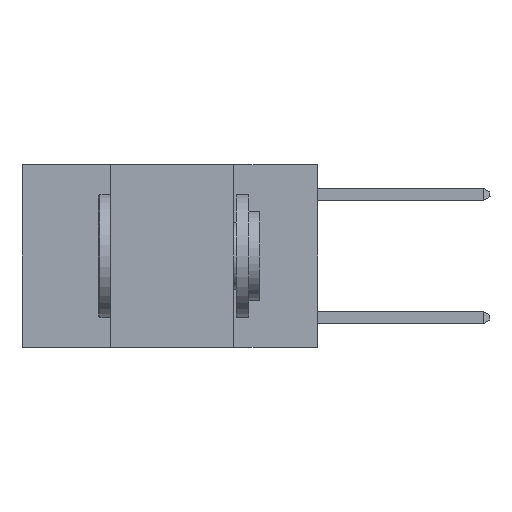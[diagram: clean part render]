
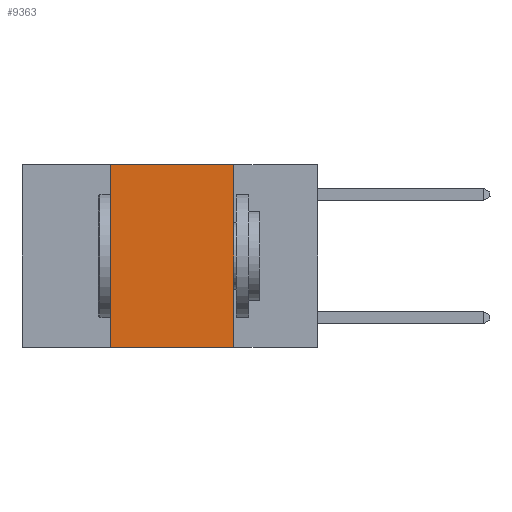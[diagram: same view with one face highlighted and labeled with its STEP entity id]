
A CAD part, left-side view. The second image highlights one B-rep face of the part: STEP entity #9363.
In plain terms, the highlighted planar face has unit normal (-1, 0, 0).
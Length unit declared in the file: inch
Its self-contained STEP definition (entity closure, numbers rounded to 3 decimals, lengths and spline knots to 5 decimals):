
#421 = DIRECTION ( 'NONE',  ( 0., 0., -1. ) ) ;
#460 = ORIENTED_EDGE ( 'NONE', *, *, #572, .F. ) ;
#572 = EDGE_CURVE ( 'NONE', #6092, #12067, #3695, .T. ) ;
#1472 = LINE ( 'NONE', #5365, #6991 ) ;
#2053 = CARTESIAN_POINT ( 'NONE',  ( 0., 0.17, -0.37 ) ) ;
#2144 = PLANE ( 'NONE',  #12619 ) ;
#2571 = LINE ( 'NONE', #11408, #7800 ) ;
#3351 = VECTOR ( 'NONE', #421, 39.37008 ) ;
#3398 = VERTEX_POINT ( 'NONE', #11470 ) ;
#3695 = LINE ( 'NONE', #10714, #3351 ) ;
#4326 = DIRECTION ( 'NONE',  ( 1., 0., 0. ) ) ;
#5365 = CARTESIAN_POINT ( 'NONE',  ( 0., 0.42, 0. ) ) ;
#5395 = CARTESIAN_POINT ( 'NONE',  ( 0., 0.6, 0. ) ) ;
#5823 = DIRECTION ( 'NONE',  ( 0., -1., 0. ) ) ;
#6092 = VERTEX_POINT ( 'NONE', #9779 ) ;
#6991 = VECTOR ( 'NONE', #14229, 39.37008 ) ;
#7011 = CARTESIAN_POINT ( 'NONE',  ( 0., 0.42, 0. ) ) ;
#7800 = VECTOR ( 'NONE', #5823, 39.37008 ) ;
#8449 = EDGE_LOOP ( 'NONE', ( #460, #9963, #9707, #10743 ) ) ;
#8505 = EDGE_CURVE ( 'NONE', #3398, #10678, #1472, .T. ) ;
#8851 = LINE ( 'NONE', #12015, #11480 ) ;
#9363 = ADVANCED_FACE ( 'NONE', ( #12208 ), #2144, .F. ) ;
#9707 = ORIENTED_EDGE ( 'NONE', *, *, #8505, .F. ) ;
#9708 = EDGE_CURVE ( 'NONE', #10678, #6092, #8851, .T. ) ;
#9779 = CARTESIAN_POINT ( 'NONE',  ( 0., 0.17, 0. ) ) ;
#9963 = ORIENTED_EDGE ( 'NONE', *, *, #9708, .F. ) ;
#10678 = VERTEX_POINT ( 'NONE', #7011 ) ;
#10714 = CARTESIAN_POINT ( 'NONE',  ( 0., 0.17, 0. ) ) ;
#10743 = ORIENTED_EDGE ( 'NONE', *, *, #12859, .T. ) ;
#10903 = DIRECTION ( 'NONE',  ( 0., -1., 0. ) ) ;
#11408 = CARTESIAN_POINT ( 'NONE',  ( 0., 0.6, -0.37 ) ) ;
#11470 = CARTESIAN_POINT ( 'NONE',  ( 0., 0.42, -0.37 ) ) ;
#11480 = VECTOR ( 'NONE', #10903, 39.37008 ) ;
#12015 = CARTESIAN_POINT ( 'NONE',  ( 0., 0.6, 0. ) ) ;
#12067 = VERTEX_POINT ( 'NONE', #2053 ) ;
#12185 = DIRECTION ( 'NONE',  ( 0., 0., -1. ) ) ;
#12208 = FACE_OUTER_BOUND ( 'NONE', #8449, .T. ) ;
#12619 = AXIS2_PLACEMENT_3D ( 'NONE', #5395, #4326, #12185 ) ;
#12859 = EDGE_CURVE ( 'NONE', #3398, #12067, #2571, .T. ) ;
#14229 = DIRECTION ( 'NONE',  ( 0., 0., 1. ) ) ;
